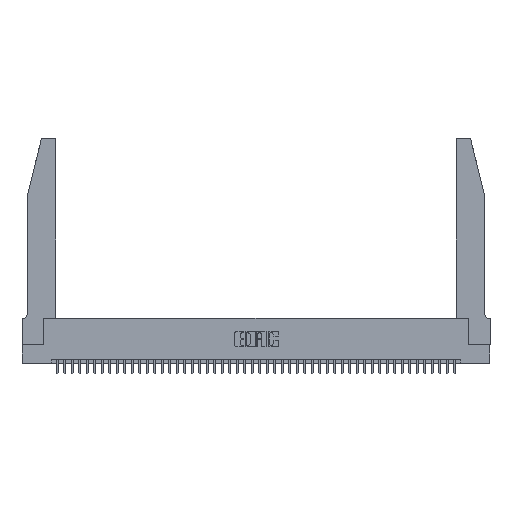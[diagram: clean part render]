
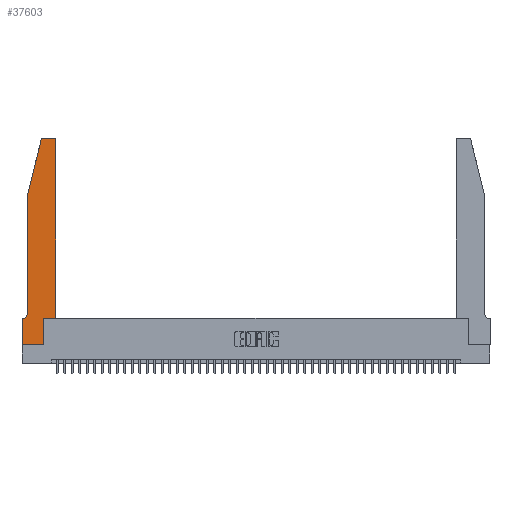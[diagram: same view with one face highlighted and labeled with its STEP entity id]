
A CAD part, top view. The second image highlights one B-rep face of the part: STEP entity #37603.
In plain terms, the highlighted planar face has unit normal (0, 0, 1).
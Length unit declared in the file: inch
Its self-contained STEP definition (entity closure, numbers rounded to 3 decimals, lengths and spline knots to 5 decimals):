
#835 = AXIS2_PLACEMENT_3D ( 'NONE', #13471, #17070, #41529 ) ;
#941 = LINE ( 'NONE', #30446, #38384 ) ;
#1470 = LINE ( 'NONE', #17988, #12005 ) ;
#1696 = VECTOR ( 'NONE', #32429, 39.37008 ) ;
#1884 = CIRCLE ( 'NONE', #5187, 0.07 ) ;
#1922 = ORIENTED_EDGE ( 'NONE', *, *, #12694, .T. ) ;
#2517 = VERTEX_POINT ( 'NONE', #36949 ) ;
#2587 = ORIENTED_EDGE ( 'NONE', *, *, #3673, .T. ) ;
#3673 = EDGE_CURVE ( 'NONE', #22049, #22687, #40744, .T. ) ;
#3898 = LINE ( 'NONE', #17069, #21634 ) ;
#4142 = VECTOR ( 'NONE', #39471, 39.37008 ) ;
#5187 = AXIS2_PLACEMENT_3D ( 'NONE', #41001, #20082, #44529 ) ;
#6308 = ORIENTED_EDGE ( 'NONE', *, *, #43206, .T. ) ;
#6810 = ORIENTED_EDGE ( 'NONE', *, *, #32755, .T. ) ;
#7378 = DIRECTION ( 'NONE',  ( 0., 0., 1. ) ) ;
#8574 = VECTOR ( 'NONE', #43172, 39.37008 ) ;
#9254 = CARTESIAN_POINT ( 'NONE',  ( 0.284, 2.72, 0.37 ) ) ;
#9635 = CARTESIAN_POINT ( 'NONE',  ( 0.2865, 0.35, 0.37 ) ) ;
#9958 = EDGE_CURVE ( 'NONE', #42399, #22049, #29867, .T. ) ;
#11495 = VERTEX_POINT ( 'NONE', #27874 ) ;
#11691 = VERTEX_POINT ( 'NONE', #14940 ) ;
#11857 = EDGE_CURVE ( 'NONE', #22687, #14366, #1470, .T. ) ;
#12005 = VECTOR ( 'NONE', #38910, 39.37008 ) ;
#12694 = EDGE_CURVE ( 'NONE', #34902, #11691, #25178, .T. ) ;
#12734 = DIRECTION ( 'NONE',  ( 0., -1., 0. ) ) ;
#12775 = CARTESIAN_POINT ( 'NONE',  ( 0.2865, 0., 0.37 ) ) ;
#12827 = DIRECTION ( 'NONE',  ( 1., 0., 0. ) ) ;
#12951 = CARTESIAN_POINT ( 'NONE',  ( 0.284, 2.75, 0.37 ) ) ;
#13024 = ORIENTED_EDGE ( 'NONE', *, *, #11857, .T. ) ;
#13423 = ORIENTED_EDGE ( 'NONE', *, *, #33051, .T. ) ;
#13471 = CARTESIAN_POINT ( 'NONE',  ( 0., 0.35, 0.37 ) ) ;
#14366 = VERTEX_POINT ( 'NONE', #41650 ) ;
#14731 = CIRCLE ( 'NONE', #25824, 0.03 ) ;
#14818 = ORIENTED_EDGE ( 'NONE', *, *, #35201, .T. ) ;
#14940 = CARTESIAN_POINT ( 'NONE',  ( 0., 0.35, 0.37 ) ) ;
#15151 = ORIENTED_EDGE ( 'NONE', *, *, #31598, .T. ) ;
#16644 = EDGE_LOOP ( 'NONE', ( #23505, #20814, #14818, #15151, #13423, #1922, #6810, #6308, #21912, #2587, #13024, #35483 ) ) ;
#16668 = LINE ( 'NONE', #21136, #43497 ) ;
#17069 = CARTESIAN_POINT ( 'NONE',  ( 0., 0., 0.37 ) ) ;
#17070 = DIRECTION ( 'NONE',  ( 0., 0., 1. ) ) ;
#17988 = CARTESIAN_POINT ( 'NONE',  ( 0.4505, 0.35, 0.37 ) ) ;
#18446 = DIRECTION ( 'NONE',  ( 1., 0., 0. ) ) ;
#18766 = CARTESIAN_POINT ( 'NONE',  ( 0.25487, 2.72718, 0.37 ) ) ;
#18786 = FACE_OUTER_BOUND ( 'NONE', #16644, .T. ) ;
#18977 = EDGE_CURVE ( 'NONE', #14366, #11495, #14731, .T. ) ;
#19778 = CARTESIAN_POINT ( 'NONE',  ( 0.2605, 2.75, 0.37 ) ) ;
#20082 = DIRECTION ( 'NONE',  ( 0., 0., -1. ) ) ;
#20814 = ORIENTED_EDGE ( 'NONE', *, *, #32183, .T. ) ;
#21057 = VECTOR ( 'NONE', #18446, 39.37008 ) ;
#21136 = CARTESIAN_POINT ( 'NONE',  ( 0.0755, 2., 0.37 ) ) ;
#21634 = VECTOR ( 'NONE', #45072, 39.37008 ) ;
#21828 = LINE ( 'NONE', #19778, #30059 ) ;
#21912 = ORIENTED_EDGE ( 'NONE', *, *, #9958, .T. ) ;
#22049 = VERTEX_POINT ( 'NONE', #9635 ) ;
#22079 = CARTESIAN_POINT ( 'NONE',  ( 0.0755, 0.35, 0.37 ) ) ;
#22315 = CARTESIAN_POINT ( 'NONE',  ( 0., 0., 0.37 ) ) ;
#22687 = VERTEX_POINT ( 'NONE', #37369 ) ;
#23315 = DIRECTION ( 'NONE',  ( -1., 0., 0. ) ) ;
#23505 = ORIENTED_EDGE ( 'NONE', *, *, #33029, .T. ) ;
#24052 = VERTEX_POINT ( 'NONE', #12951 ) ;
#24676 = DIRECTION ( 'NONE',  ( -0.239, -0.971, 0. ) ) ;
#25178 = LINE ( 'NONE', #22079, #4142 ) ;
#25719 = CARTESIAN_POINT ( 'NONE',  ( 0.2865, 0.35, 0.37 ) ) ;
#25824 = AXIS2_PLACEMENT_3D ( 'NONE', #28524, #7378, #32044 ) ;
#27874 = CARTESIAN_POINT ( 'NONE',  ( 0.4205, 2.75, 0.37 ) ) ;
#28524 = CARTESIAN_POINT ( 'NONE',  ( 0.4205, 2.72, 0.37 ) ) ;
#28927 = VERTEX_POINT ( 'NONE', #22315 ) ;
#29867 = LINE ( 'NONE', #25719, #1696 ) ;
#30055 = CARTESIAN_POINT ( 'NONE',  ( 0.0055, 0.35, 0.37 ) ) ;
#30059 = VECTOR ( 'NONE', #23315, 39.37008 ) ;
#30446 = CARTESIAN_POINT ( 'NONE',  ( 0.0755, 2., 0.37 ) ) ;
#31598 = EDGE_CURVE ( 'NONE', #2517, #44190, #941, .T. ) ;
#32029 = VERTEX_POINT ( 'NONE', #18766 ) ;
#32044 = DIRECTION ( 'NONE',  ( 1., 0., 0. ) ) ;
#32183 = EDGE_CURVE ( 'NONE', #24052, #32029, #41061, .T. ) ;
#32429 = DIRECTION ( 'NONE',  ( 0., 1., 0. ) ) ;
#32755 = EDGE_CURVE ( 'NONE', #11691, #28927, #35525, .T. ) ;
#33029 = EDGE_CURVE ( 'NONE', #11495, #24052, #21828, .T. ) ;
#33051 = EDGE_CURVE ( 'NONE', #44190, #34902, #1884, .T. ) ;
#33803 = AXIS2_PLACEMENT_3D ( 'NONE', #9254, #33883, #12827 ) ;
#33883 = DIRECTION ( 'NONE',  ( 0., 0., 1. ) ) ;
#34526 = PLANE ( 'NONE',  #835 ) ;
#34902 = VERTEX_POINT ( 'NONE', #30055 ) ;
#35201 = EDGE_CURVE ( 'NONE', #32029, #2517, #16668, .T. ) ;
#35483 = ORIENTED_EDGE ( 'NONE', *, *, #18977, .T. ) ;
#35525 = LINE ( 'NONE', #39637, #8574 ) ;
#36949 = CARTESIAN_POINT ( 'NONE',  ( 0.0755, 2., 0.37 ) ) ;
#37369 = CARTESIAN_POINT ( 'NONE',  ( 0.4505, 0.35, 0.37 ) ) ;
#37603 = ADVANCED_FACE ( 'NONE', ( #18786 ), #34526, .T. ) ;
#38384 = VECTOR ( 'NONE', #12734, 39.37008 ) ;
#38910 = DIRECTION ( 'NONE',  ( 0., 1., 0. ) ) ;
#39360 = CARTESIAN_POINT ( 'NONE',  ( 0.4505, 0.35, 0.37 ) ) ;
#39471 = DIRECTION ( 'NONE',  ( -1., 0., 0. ) ) ;
#39612 = CARTESIAN_POINT ( 'NONE',  ( 0.0755, 0.42, 0.37 ) ) ;
#39637 = CARTESIAN_POINT ( 'NONE',  ( 0., 0., 0.37 ) ) ;
#40744 = LINE ( 'NONE', #39360, #21057 ) ;
#41001 = CARTESIAN_POINT ( 'NONE',  ( 0.0055, 0.42, 0.37 ) ) ;
#41061 = CIRCLE ( 'NONE', #33803, 0.03 ) ;
#41529 = DIRECTION ( 'NONE',  ( 1., 0., 0. ) ) ;
#41650 = CARTESIAN_POINT ( 'NONE',  ( 0.4505, 2.72, 0.37 ) ) ;
#42399 = VERTEX_POINT ( 'NONE', #12775 ) ;
#43172 = DIRECTION ( 'NONE',  ( 0., -1., 0. ) ) ;
#43206 = EDGE_CURVE ( 'NONE', #28927, #42399, #3898, .T. ) ;
#43497 = VECTOR ( 'NONE', #24676, 39.37008 ) ;
#44190 = VERTEX_POINT ( 'NONE', #39612 ) ;
#44529 = DIRECTION ( 'NONE',  ( -1., 0., 0. ) ) ;
#45072 = DIRECTION ( 'NONE',  ( 1., 0., 0. ) ) ;
